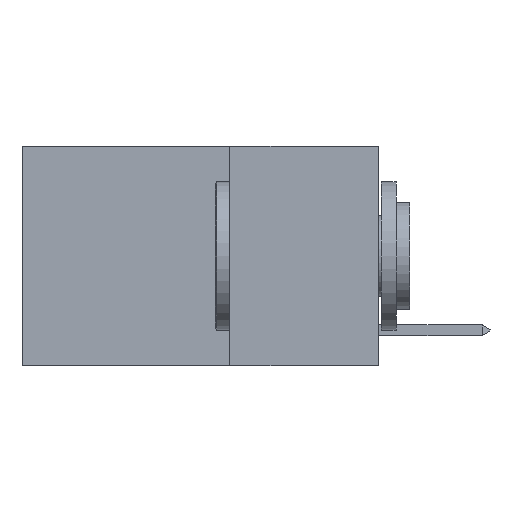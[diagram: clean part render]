
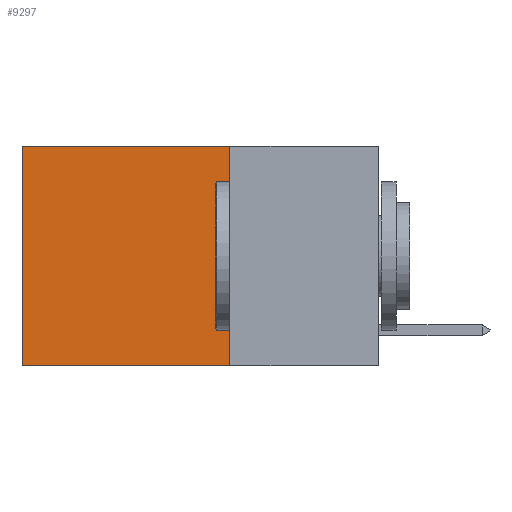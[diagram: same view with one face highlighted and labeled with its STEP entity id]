
A CAD part, left-side view. The second image highlights one B-rep face of the part: STEP entity #9297.
In plain terms, the highlighted planar face has unit normal (-1, 0, 0).
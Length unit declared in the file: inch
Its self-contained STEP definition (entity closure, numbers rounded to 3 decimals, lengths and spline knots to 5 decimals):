
#1684 = EDGE_LOOP ( 'NONE', ( #8839, #17584, #6161, #20141 ) ) ;
#1868 = EDGE_CURVE ( 'NONE', #7109, #15457, #19364, .T. ) ;
#3174 = VECTOR ( 'NONE', #20471, 39.37008 ) ;
#4710 = VECTOR ( 'NONE', #17423, 39.37008 ) ;
#5537 = EDGE_CURVE ( 'NONE', #7109, #19275, #23280, .T. ) ;
#5736 = DIRECTION ( 'NONE',  ( 0., 0., -1. ) ) ;
#6150 = CARTESIAN_POINT ( 'NONE',  ( 0.2625, 0.25, 0. ) ) ;
#6161 = ORIENTED_EDGE ( 'NONE', *, *, #1868, .F. ) ;
#6494 = CARTESIAN_POINT ( 'NONE',  ( 0.2625, 0.25, 0. ) ) ;
#7109 = VERTEX_POINT ( 'NONE', #23374 ) ;
#7455 = CARTESIAN_POINT ( 'NONE',  ( 0.2625, 0.25, -0.37 ) ) ;
#7980 = DIRECTION ( 'NONE',  ( 1., 0., 0. ) ) ;
#8090 = LINE ( 'NONE', #18701, #3174 ) ;
#8839 = ORIENTED_EDGE ( 'NONE', *, *, #14289, .T. ) ;
#8977 = CARTESIAN_POINT ( 'NONE',  ( 0.2625, 0.6, -0.37 ) ) ;
#9297 = ADVANCED_FACE ( 'NONE', ( #17322 ), #18825, .F. ) ;
#9340 = CARTESIAN_POINT ( 'NONE',  ( 0.2625, 0.6, 0. ) ) ;
#9457 = DIRECTION ( 'NONE',  ( 0., 0., -1. ) ) ;
#9709 = CARTESIAN_POINT ( 'NONE',  ( 0.2625, 0.25, 0. ) ) ;
#11179 = AXIS2_PLACEMENT_3D ( 'NONE', #6150, #7980, #20596 ) ;
#11356 = LINE ( 'NONE', #9340, #20336 ) ;
#11534 = EDGE_CURVE ( 'NONE', #15457, #21726, #8090, .T. ) ;
#12454 = CARTESIAN_POINT ( 'NONE',  ( 0.2625, 0.6, 0. ) ) ;
#14289 = EDGE_CURVE ( 'NONE', #19275, #21726, #11356, .T. ) ;
#14619 = VECTOR ( 'NONE', #9457, 39.37008 ) ;
#15457 = VERTEX_POINT ( 'NONE', #7455 ) ;
#17322 = FACE_OUTER_BOUND ( 'NONE', #1684, .T. ) ;
#17423 = DIRECTION ( 'NONE',  ( 0., 1., 0. ) ) ;
#17584 = ORIENTED_EDGE ( 'NONE', *, *, #11534, .F. ) ;
#18701 = CARTESIAN_POINT ( 'NONE',  ( 0.2625, 0.25, -0.37 ) ) ;
#18825 = PLANE ( 'NONE',  #11179 ) ;
#19275 = VERTEX_POINT ( 'NONE', #12454 ) ;
#19364 = LINE ( 'NONE', #9709, #14619 ) ;
#20141 = ORIENTED_EDGE ( 'NONE', *, *, #5537, .T. ) ;
#20336 = VECTOR ( 'NONE', #5736, 39.37008 ) ;
#20471 = DIRECTION ( 'NONE',  ( 0., 1., 0. ) ) ;
#20596 = DIRECTION ( 'NONE',  ( 0., 0., -1. ) ) ;
#21726 = VERTEX_POINT ( 'NONE', #8977 ) ;
#23280 = LINE ( 'NONE', #6494, #4710 ) ;
#23374 = CARTESIAN_POINT ( 'NONE',  ( 0.2625, 0.25, 0. ) ) ;
